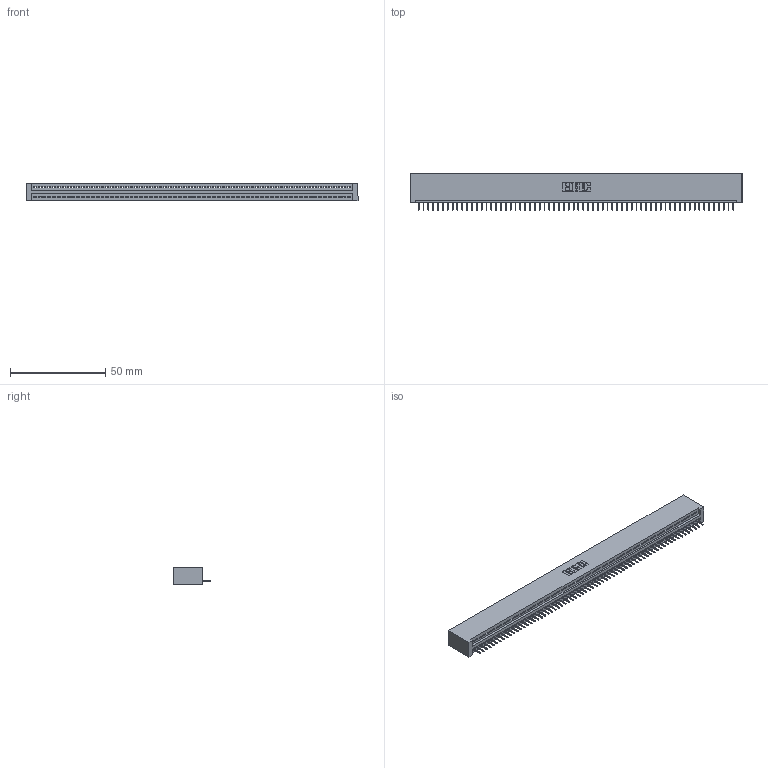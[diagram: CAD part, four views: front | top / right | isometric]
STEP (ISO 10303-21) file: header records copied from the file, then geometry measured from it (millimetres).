
FILE_DESCRIPTION (( 'STEP AP203' ), '1' );
FILE_NAME ('345-066-524-101.STEP', '2019-10-11T21:06:34', ( '' ), ( '' ), 'SwSTEP 2.0', 'SolidWorks 2016', '' );
FILE_SCHEMA (( 'CONFIG_CONTROL_DESIGN' ));
Length unit declared in the file: inch
Products named in the file (3): 345-292-001_345-293-124; 345 Part_No Mounting Lugs; 345-066-524-101
Assembly tree (67 placements, depth 2):
  345-066-524-101
    345 Part_No Mounting Lugs
    345-292-001_345-293-124  x66
Bounding box: 174.24 x 19.35 x 9.4 mm (x, y, z)
Volume: 17070.1 mm3; surface area: 22367.3 mm2
Topology: 67 solids, 67 shells, 4210 faces, 12197 edges, 7866 vertices
Faces by surface type: plane 3112, cylinder 1098
Entity records: 46239 total; most frequent: ORIENTED_EDGE 8014, CARTESIAN_POINT 8014, DIRECTION 6959, EDGE_CURVE 4007, LINE 3623, VECTOR 3623, VERTEX_POINT 2666, AXIS2_PLACEMENT_3D 1668
